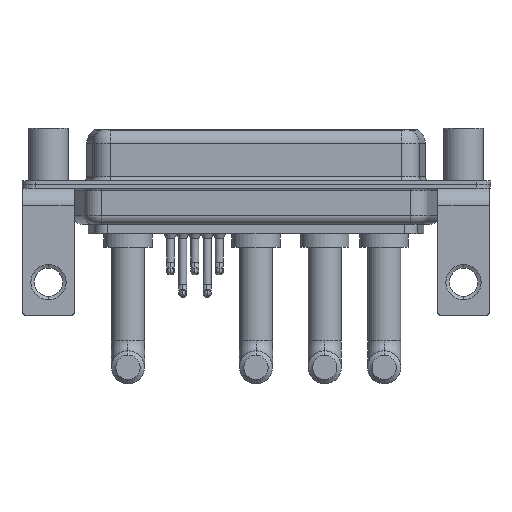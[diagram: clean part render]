
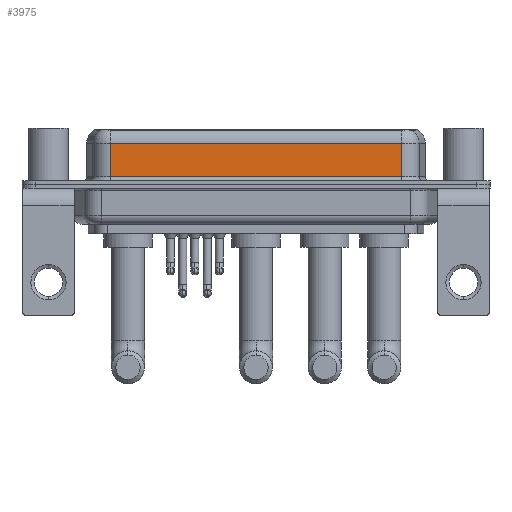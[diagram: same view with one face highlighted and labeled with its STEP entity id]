
A CAD part, front view. The second image highlights one B-rep face of the part: STEP entity #3975.
In plain terms, the highlighted planar face has unit normal (0, -1, 0).
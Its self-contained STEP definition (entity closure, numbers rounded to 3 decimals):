
#705 = EDGE_CURVE ( 'NONE', #6212, #17776, #11171, .T. ) ;
#968 = ORIENTED_EDGE ( 'NONE', *, *, #705, .F. ) ;
#1599 = DIRECTION ( 'NONE',  ( 0., 0., -1. ) ) ;
#3140 = CARTESIAN_POINT ( 'NONE',  ( 40.037, -3.95, 4.65 ) ) ;
#3762 = CARTESIAN_POINT ( 'NONE',  ( 7.013, -3.95, 4.65 ) ) ;
#3943 = ORIENTED_EDGE ( 'NONE', *, *, #5249, .T. ) ;
#3975 = ADVANCED_FACE ( 'NONE', ( #12896 ), #6864, .F. ) ;
#5249 = EDGE_CURVE ( 'NONE', #15685, #6535, #6245, .T. ) ;
#5358 = DIRECTION ( 'NONE',  ( 0., 1., 0. ) ) ;
#5773 = VECTOR ( 'NONE', #9573, 1000. ) ;
#6212 = VERTEX_POINT ( 'NONE', #3140 ) ;
#6245 = LINE ( 'NONE', #16993, #6619 ) ;
#6459 = DIRECTION ( 'NONE',  ( -1., 0., 0. ) ) ;
#6535 = VERTEX_POINT ( 'NONE', #12681 ) ;
#6619 = VECTOR ( 'NONE', #1599, 1000. ) ;
#6864 = PLANE ( 'NONE',  #10056 ) ;
#7297 = CARTESIAN_POINT ( 'NONE',  ( 40.037, -3.95, 0.9 ) ) ;
#9028 = ORIENTED_EDGE ( 'NONE', *, *, #9112, .T. ) ;
#9110 = DIRECTION ( 'NONE',  ( 1., 0., 0. ) ) ;
#9112 = EDGE_CURVE ( 'NONE', #6535, #17776, #10309, .T. ) ;
#9573 = DIRECTION ( 'NONE',  ( 0., 0., -1. ) ) ;
#10056 = AXIS2_PLACEMENT_3D ( 'NONE', #15806, #5358, #19029 ) ;
#10309 = LINE ( 'NONE', #7297, #18555 ) ;
#10406 = ORIENTED_EDGE ( 'NONE', *, *, #12942, .T. ) ;
#11171 = LINE ( 'NONE', #14373, #5773 ) ;
#11185 = LINE ( 'NONE', #17603, #15445 ) ;
#12681 = CARTESIAN_POINT ( 'NONE',  ( 7.013, -3.95, 0.9 ) ) ;
#12896 = FACE_OUTER_BOUND ( 'NONE', #15648, .T. ) ;
#12942 = EDGE_CURVE ( 'NONE', #6212, #15685, #11185, .T. ) ;
#14046 = CARTESIAN_POINT ( 'NONE',  ( 40.037, -3.95, 0.9 ) ) ;
#14373 = CARTESIAN_POINT ( 'NONE',  ( 40.037, -3.95, 6.4 ) ) ;
#15445 = VECTOR ( 'NONE', #6459, 1000. ) ;
#15648 = EDGE_LOOP ( 'NONE', ( #968, #10406, #3943, #9028 ) ) ;
#15685 = VERTEX_POINT ( 'NONE', #3762 ) ;
#15806 = CARTESIAN_POINT ( 'NONE',  ( 40.037, -3.95, 6.4 ) ) ;
#16993 = CARTESIAN_POINT ( 'NONE',  ( 7.013, -3.95, 6.4 ) ) ;
#17603 = CARTESIAN_POINT ( 'NONE',  ( 40.037, -3.95, 4.65 ) ) ;
#17776 = VERTEX_POINT ( 'NONE', #14046 ) ;
#18555 = VECTOR ( 'NONE', #9110, 1000. ) ;
#19029 = DIRECTION ( 'NONE',  ( 0., 0., 1. ) ) ;
